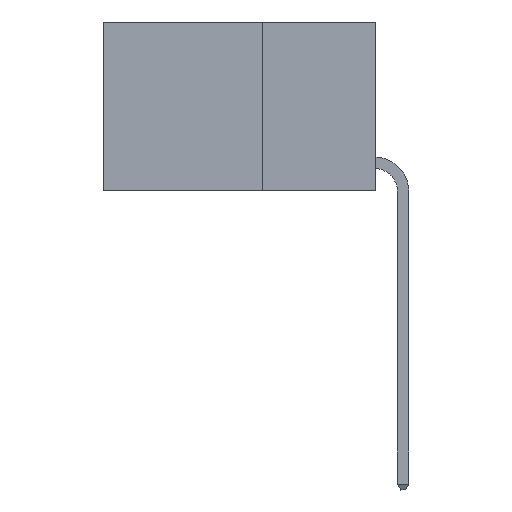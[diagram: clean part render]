
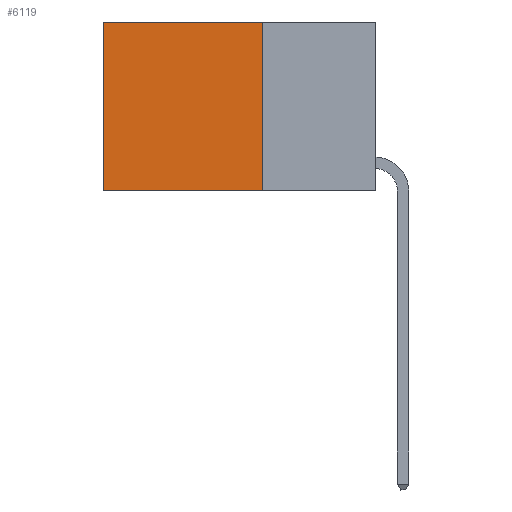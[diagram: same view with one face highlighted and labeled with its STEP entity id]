
A CAD part, left-side view. The second image highlights one B-rep face of the part: STEP entity #6119.
In plain terms, the highlighted planar face has unit normal (-1, 0, 0).
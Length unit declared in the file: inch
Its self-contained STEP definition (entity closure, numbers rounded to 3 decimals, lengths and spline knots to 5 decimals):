
#327 = CARTESIAN_POINT ( 'NONE',  ( 0.2625, 0.25, -0.37 ) ) ;
#442 = CARTESIAN_POINT ( 'NONE',  ( 0.2625, 0.25, 0. ) ) ;
#909 = CARTESIAN_POINT ( 'NONE',  ( 0.2625, 0.6, 0. ) ) ;
#1714 = EDGE_CURVE ( 'NONE', #24381, #25471, #4848, .T. ) ;
#2289 = PLANE ( 'NONE',  #18248 ) ;
#2851 = VERTEX_POINT ( 'NONE', #442 ) ;
#4029 = VECTOR ( 'NONE', #15813, 39.37008 ) ;
#4848 = LINE ( 'NONE', #19102, #20249 ) ;
#6119 = ADVANCED_FACE ( 'NONE', ( #10719 ), #2289, .F. ) ;
#6514 = LINE ( 'NONE', #15091, #16253 ) ;
#7178 = DIRECTION ( 'NONE',  ( 0., 1., 0. ) ) ;
#7652 = EDGE_CURVE ( 'NONE', #2851, #24847, #22470, .T. ) ;
#8626 = CARTESIAN_POINT ( 'NONE',  ( 0.2625, 0.6, -0.37 ) ) ;
#10719 = FACE_OUTER_BOUND ( 'NONE', #26371, .T. ) ;
#11948 = CARTESIAN_POINT ( 'NONE',  ( 0.2625, 0.25, 0. ) ) ;
#12922 = CARTESIAN_POINT ( 'NONE',  ( 0.2625, 0.25, 0. ) ) ;
#13536 = CARTESIAN_POINT ( 'NONE',  ( 0.2625, 0.25, 0. ) ) ;
#14158 = ORIENTED_EDGE ( 'NONE', *, *, #24778, .F. ) ;
#15091 = CARTESIAN_POINT ( 'NONE',  ( 0.2625, 0.25, -0.37 ) ) ;
#15261 = DIRECTION ( 'NONE',  ( 1., 0., 0. ) ) ;
#15713 = VECTOR ( 'NONE', #7178, 39.37008 ) ;
#15813 = DIRECTION ( 'NONE',  ( 0., 0., -1. ) ) ;
#16188 = ORIENTED_EDGE ( 'NONE', *, *, #1714, .T. ) ;
#16253 = VECTOR ( 'NONE', #23561, 39.37008 ) ;
#18248 = AXIS2_PLACEMENT_3D ( 'NONE', #12922, #15261, #19157 ) ;
#18720 = ORIENTED_EDGE ( 'NONE', *, *, #7652, .F. ) ;
#19102 = CARTESIAN_POINT ( 'NONE',  ( 0.2625, 0.6, 0. ) ) ;
#19157 = DIRECTION ( 'NONE',  ( 0., 0., -1. ) ) ;
#20036 = EDGE_CURVE ( 'NONE', #2851, #24381, #22909, .T. ) ;
#20141 = ORIENTED_EDGE ( 'NONE', *, *, #20036, .T. ) ;
#20249 = VECTOR ( 'NONE', #21584, 39.37008 ) ;
#21584 = DIRECTION ( 'NONE',  ( 0., 0., -1. ) ) ;
#22470 = LINE ( 'NONE', #11948, #4029 ) ;
#22909 = LINE ( 'NONE', #13536, #15713 ) ;
#23561 = DIRECTION ( 'NONE',  ( 0., 1., 0. ) ) ;
#24381 = VERTEX_POINT ( 'NONE', #909 ) ;
#24778 = EDGE_CURVE ( 'NONE', #24847, #25471, #6514, .T. ) ;
#24847 = VERTEX_POINT ( 'NONE', #327 ) ;
#25471 = VERTEX_POINT ( 'NONE', #8626 ) ;
#26371 = EDGE_LOOP ( 'NONE', ( #16188, #14158, #18720, #20141 ) ) ;
